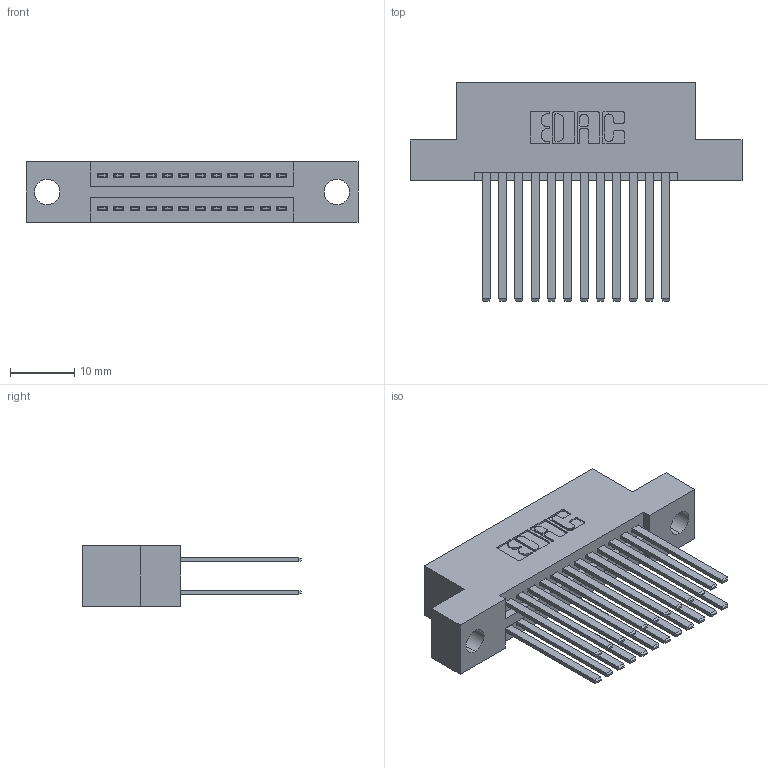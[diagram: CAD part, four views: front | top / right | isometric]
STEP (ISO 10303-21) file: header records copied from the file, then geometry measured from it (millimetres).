
FILE_DESCRIPTION (( 'STEP AP203' ), '1' );
FILE_NAME ('395-024-544-204.STEP', '2021-06-16T19:14:04', ( '' ), ( '' ), 'SwSTEP 2.0', 'SolidWorks 2020', '' );
FILE_SCHEMA (( 'CONFIG_CONTROL_DESIGN' ));
Length unit declared in the file: inch
Products named in the file (3): 395-024-544-204; 345 Part_Flush Mounting Lugs - 0.156 Dia-TI; 345-292-001_345-293-144
Assembly tree (25 placements, depth 2):
  395-024-544-204
    345 Part_Flush Mounting Lugs - 0.156 Dia-TI
    345-292-001_345-293-144  x24
Bounding box: 51.69 x 33.96 x 9.4 mm (x, y, z)
Volume: 4973.1 mm3; surface area: 7607.8 mm2
Topology: 25 solids, 25 shells, 1196 faces, 3521 edges, 2314 vertices
Faces by surface type: plane 790, cylinder 406
Entity records: 13689 total; most frequent: CARTESIAN_POINT 2326, ORIENTED_EDGE 2258, DIRECTION 2085, EDGE_CURVE 1129, LINE 953, VECTOR 953, VERTEX_POINT 750, AXIS2_PLACEMENT_3D 566
